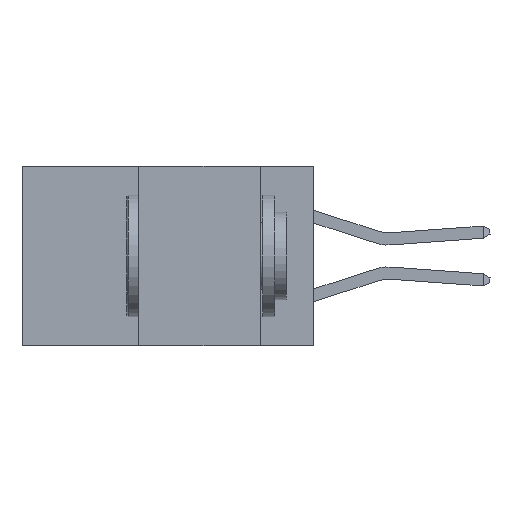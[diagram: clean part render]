
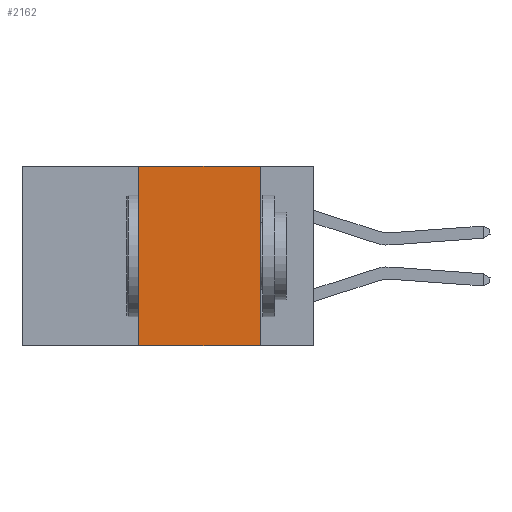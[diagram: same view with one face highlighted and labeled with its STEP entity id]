
A CAD part, left-side view. The second image highlights one B-rep face of the part: STEP entity #2162.
In plain terms, the highlighted planar face has unit normal (-1, 0, 0).
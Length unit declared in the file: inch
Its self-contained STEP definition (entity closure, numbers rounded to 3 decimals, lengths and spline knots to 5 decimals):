
#60 = VERTEX_POINT ( 'NONE', #7005 ) ;
#204 = CARTESIAN_POINT ( 'NONE',  ( 0., 0.6, 0. ) ) ;
#236 = CARTESIAN_POINT ( 'NONE',  ( 0., 0.11, 0. ) ) ;
#346 = VECTOR ( 'NONE', #3428, 39.37008 ) ;
#718 = ORIENTED_EDGE ( 'NONE', *, *, #6626, .F. ) ;
#733 = EDGE_LOOP ( 'NONE', ( #718, #860, #1076, #1538 ) ) ;
#860 = ORIENTED_EDGE ( 'NONE', *, *, #7815, .F. ) ;
#1076 = ORIENTED_EDGE ( 'NONE', *, *, #5179, .F. ) ;
#1272 = LINE ( 'NONE', #236, #6410 ) ;
#1533 = FACE_OUTER_BOUND ( 'NONE', #733, .T. ) ;
#1538 = ORIENTED_EDGE ( 'NONE', *, *, #6313, .T. ) ;
#1935 = LINE ( 'NONE', #204, #8044 ) ;
#2162 = ADVANCED_FACE ( 'NONE', ( #1533 ), #6223, .F. ) ;
#2225 = CARTESIAN_POINT ( 'NONE',  ( 0., 0.36, 0. ) ) ;
#2922 = DIRECTION ( 'NONE',  ( 0., 0., 1. ) ) ;
#3255 = LINE ( 'NONE', #4812, #346 ) ;
#3346 = DIRECTION ( 'NONE',  ( 0., 0., -1. ) ) ;
#3428 = DIRECTION ( 'NONE',  ( 0., -1., 0. ) ) ;
#4812 = CARTESIAN_POINT ( 'NONE',  ( 0., 0.6, -0.37 ) ) ;
#4857 = VECTOR ( 'NONE', #2922, 39.37008 ) ;
#4900 = CARTESIAN_POINT ( 'NONE',  ( 0., 0.11, -0.37 ) ) ;
#5078 = VERTEX_POINT ( 'NONE', #5103 ) ;
#5083 = AXIS2_PLACEMENT_3D ( 'NONE', #7854, #10282, #8588 ) ;
#5103 = CARTESIAN_POINT ( 'NONE',  ( 0., 0.36, 0. ) ) ;
#5179 = EDGE_CURVE ( 'NONE', #6622, #5078, #7488, .T. ) ;
#5822 = DIRECTION ( 'NONE',  ( 0., -1., 0. ) ) ;
#6223 = PLANE ( 'NONE',  #5083 ) ;
#6313 = EDGE_CURVE ( 'NONE', #6622, #7173, #3255, .T. ) ;
#6410 = VECTOR ( 'NONE', #3346, 39.37008 ) ;
#6622 = VERTEX_POINT ( 'NONE', #10323 ) ;
#6626 = EDGE_CURVE ( 'NONE', #60, #7173, #1272, .T. ) ;
#7005 = CARTESIAN_POINT ( 'NONE',  ( 0., 0.11, 0. ) ) ;
#7173 = VERTEX_POINT ( 'NONE', #4900 ) ;
#7488 = LINE ( 'NONE', #2225, #4857 ) ;
#7815 = EDGE_CURVE ( 'NONE', #5078, #60, #1935, .T. ) ;
#7854 = CARTESIAN_POINT ( 'NONE',  ( 0., 0.6, 0. ) ) ;
#8044 = VECTOR ( 'NONE', #5822, 39.37008 ) ;
#8588 = DIRECTION ( 'NONE',  ( 0., 0., -1. ) ) ;
#10282 = DIRECTION ( 'NONE',  ( 1., 0., 0. ) ) ;
#10323 = CARTESIAN_POINT ( 'NONE',  ( 0., 0.36, -0.37 ) ) ;
